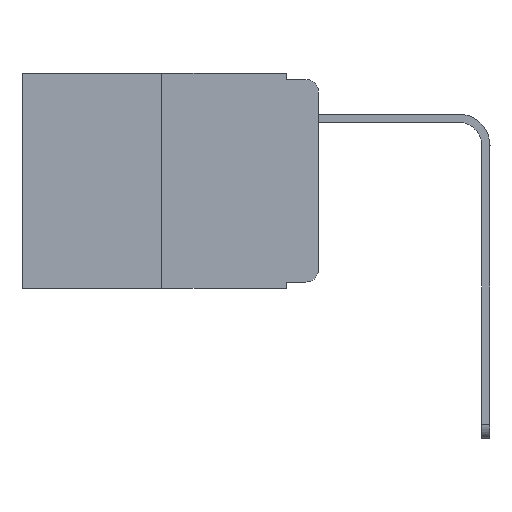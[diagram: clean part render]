
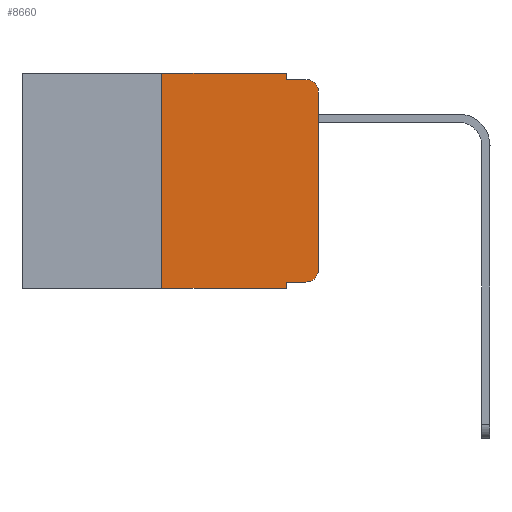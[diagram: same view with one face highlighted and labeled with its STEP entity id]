
A CAD part, left-side view. The second image highlights one B-rep face of the part: STEP entity #8660.
In plain terms, the highlighted planar face has unit normal (-1, 0, 0).
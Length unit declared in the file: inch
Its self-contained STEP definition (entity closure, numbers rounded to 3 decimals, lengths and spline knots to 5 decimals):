
#96 = EDGE_CURVE ( 'NONE', #7906, #6469, #7753, .T. ) ;
#518 = ORIENTED_EDGE ( 'NONE', *, *, #7883, .T. ) ;
#1137 = CARTESIAN_POINT ( 'NONE',  ( 0., 0.473, 0. ) ) ;
#1259 = FACE_OUTER_BOUND ( 'NONE', #1609, .T. ) ;
#1589 = DIRECTION ( 'NONE',  ( -1., 0., 0. ) ) ;
#1596 = DIRECTION ( 'NONE',  ( 0., 0., -1. ) ) ;
#1609 = EDGE_LOOP ( 'NONE', ( #518, #8549, #9088, #11809, #11029, #5946, #9658, #9136, #9779, #8130 ) ) ;
#1630 = CARTESIAN_POINT ( 'NONE',  ( 0., 0.051, 0. ) ) ;
#1696 = CARTESIAN_POINT ( 'NONE',  ( 0., 0.051, -0.333 ) ) ;
#1735 = CARTESIAN_POINT ( 'NONE',  ( 0., 0.02, -0.313 ) ) ;
#1790 = EDGE_CURVE ( 'NONE', #5393, #11966, #9548, .T. ) ;
#2137 = PLANE ( 'NONE',  #11056 ) ;
#2390 = VECTOR ( 'NONE', #3532, 39.37008 ) ;
#2508 = VECTOR ( 'NONE', #6853, 39.37008 ) ;
#2597 = CARTESIAN_POINT ( 'NONE',  ( 0., 0.02, -0.03 ) ) ;
#2725 = EDGE_CURVE ( 'NONE', #3070, #6469, #4928, .T. ) ;
#3070 = VERTEX_POINT ( 'NONE', #11880 ) ;
#3225 = LINE ( 'NONE', #12222, #9926 ) ;
#3532 = DIRECTION ( 'NONE',  ( 0., -1., 0. ) ) ;
#3966 = LINE ( 'NONE', #10431, #7845 ) ;
#4222 = CARTESIAN_POINT ( 'NONE',  ( 0., 0., -0.313 ) ) ;
#4482 = CARTESIAN_POINT ( 'NONE',  ( 0., 0.02, -0.01 ) ) ;
#4745 = LINE ( 'NONE', #1137, #2508 ) ;
#4759 = CARTESIAN_POINT ( 'NONE',  ( 0., 0.051, -0.333 ) ) ;
#4797 = EDGE_CURVE ( 'NONE', #10254, #5393, #4745, .T. ) ;
#4810 = DIRECTION ( 'NONE',  ( 0., 0., -1. ) ) ;
#4928 = LINE ( 'NONE', #6490, #2390 ) ;
#4935 = CARTESIAN_POINT ( 'NONE',  ( 0., 0.02, -0.333 ) ) ;
#4961 = CIRCLE ( 'NONE', #10742, 0.02 ) ;
#5273 = EDGE_CURVE ( 'NONE', #9134, #6466, #9783, .T. ) ;
#5393 = VERTEX_POINT ( 'NONE', #10362 ) ;
#5631 = LINE ( 'NONE', #4759, #10240 ) ;
#5773 = DIRECTION ( 'NONE',  ( 0., -1., 0. ) ) ;
#5946 = ORIENTED_EDGE ( 'NONE', *, *, #10163, .F. ) ;
#6427 = VECTOR ( 'NONE', #7593, 39.37008 ) ;
#6431 = VECTOR ( 'NONE', #1596, 39.37008 ) ;
#6466 = VERTEX_POINT ( 'NONE', #4482 ) ;
#6469 = VERTEX_POINT ( 'NONE', #6559 ) ;
#6490 = CARTESIAN_POINT ( 'NONE',  ( 0., 0.473, -0.343 ) ) ;
#6559 = CARTESIAN_POINT ( 'NONE',  ( 0., 0.051, -0.343 ) ) ;
#6614 = DIRECTION ( 'NONE',  ( 0., 0., 1. ) ) ;
#6853 = DIRECTION ( 'NONE',  ( 0., -1., 0. ) ) ;
#7469 = CARTESIAN_POINT ( 'NONE',  ( 0., 0.25, 0. ) ) ;
#7593 = DIRECTION ( 'NONE',  ( 0., 0., -1. ) ) ;
#7753 = LINE ( 'NONE', #8553, #6427 ) ;
#7812 = DIRECTION ( 'NONE',  ( 1., 0., 0. ) ) ;
#7845 = VECTOR ( 'NONE', #6614, 39.37008 ) ;
#7883 = EDGE_CURVE ( 'NONE', #9442, #9134, #3966, .T. ) ;
#7906 = VERTEX_POINT ( 'NONE', #1696 ) ;
#8107 = LINE ( 'NONE', #11531, #11217 ) ;
#8130 = ORIENTED_EDGE ( 'NONE', *, *, #11420, .T. ) ;
#8549 = ORIENTED_EDGE ( 'NONE', *, *, #5273, .T. ) ;
#8553 = CARTESIAN_POINT ( 'NONE',  ( 0., 0.051, 0. ) ) ;
#8660 = ADVANCED_FACE ( 'NONE', ( #1259 ), #2137, .F. ) ;
#9088 = ORIENTED_EDGE ( 'NONE', *, *, #9093, .F. ) ;
#9093 = EDGE_CURVE ( 'NONE', #11966, #6466, #8107, .T. ) ;
#9134 = VERTEX_POINT ( 'NONE', #11575 ) ;
#9136 = ORIENTED_EDGE ( 'NONE', *, *, #96, .F. ) ;
#9442 = VERTEX_POINT ( 'NONE', #4222 ) ;
#9548 = LINE ( 'NONE', #1630, #6431 ) ;
#9586 = CARTESIAN_POINT ( 'NONE',  ( 0., 0.473, 0. ) ) ;
#9658 = ORIENTED_EDGE ( 'NONE', *, *, #2725, .T. ) ;
#9660 = EDGE_CURVE ( 'NONE', #7906, #11994, #5631, .T. ) ;
#9779 = ORIENTED_EDGE ( 'NONE', *, *, #9660, .T. ) ;
#9783 = CIRCLE ( 'NONE', #11419, 0.02 ) ;
#9926 = VECTOR ( 'NONE', #10232, 39.37008 ) ;
#10163 = EDGE_CURVE ( 'NONE', #3070, #10254, #3225, .T. ) ;
#10230 = DIRECTION ( 'NONE',  ( -1., 0., 0. ) ) ;
#10232 = DIRECTION ( 'NONE',  ( 0., 0., 1. ) ) ;
#10240 = VECTOR ( 'NONE', #10365, 39.37008 ) ;
#10245 = DIRECTION ( 'NONE',  ( 0., 0., -1. ) ) ;
#10254 = VERTEX_POINT ( 'NONE', #7469 ) ;
#10362 = CARTESIAN_POINT ( 'NONE',  ( 0., 0.051, 0. ) ) ;
#10365 = DIRECTION ( 'NONE',  ( 0., -1., 0. ) ) ;
#10431 = CARTESIAN_POINT ( 'NONE',  ( 0., 0., 0. ) ) ;
#10742 = AXIS2_PLACEMENT_3D ( 'NONE', #1735, #10230, #11187 ) ;
#10894 = CARTESIAN_POINT ( 'NONE',  ( 0., 0.051, -0.01 ) ) ;
#11029 = ORIENTED_EDGE ( 'NONE', *, *, #4797, .F. ) ;
#11056 = AXIS2_PLACEMENT_3D ( 'NONE', #9586, #7812, #4810 ) ;
#11187 = DIRECTION ( 'NONE',  ( 0., 0., -1. ) ) ;
#11217 = VECTOR ( 'NONE', #5773, 39.37008 ) ;
#11419 = AXIS2_PLACEMENT_3D ( 'NONE', #2597, #1589, #10245 ) ;
#11420 = EDGE_CURVE ( 'NONE', #11994, #9442, #4961, .T. ) ;
#11531 = CARTESIAN_POINT ( 'NONE',  ( 0., 0.051, -0.01 ) ) ;
#11575 = CARTESIAN_POINT ( 'NONE',  ( 0., 0., -0.03 ) ) ;
#11809 = ORIENTED_EDGE ( 'NONE', *, *, #1790, .F. ) ;
#11880 = CARTESIAN_POINT ( 'NONE',  ( 0., 0.25, -0.343 ) ) ;
#11966 = VERTEX_POINT ( 'NONE', #10894 ) ;
#11994 = VERTEX_POINT ( 'NONE', #4935 ) ;
#12222 = CARTESIAN_POINT ( 'NONE',  ( 0., 0.25, 0. ) ) ;
